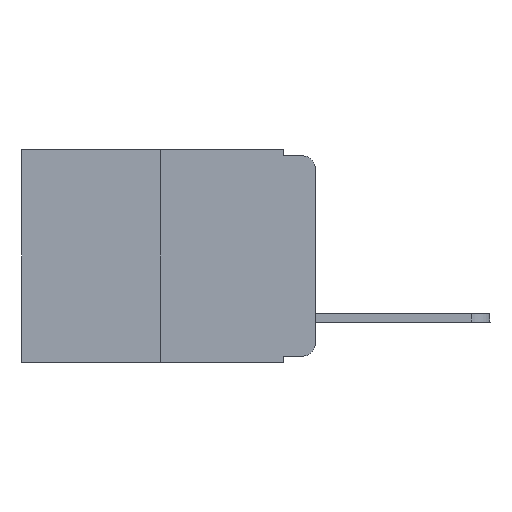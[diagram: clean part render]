
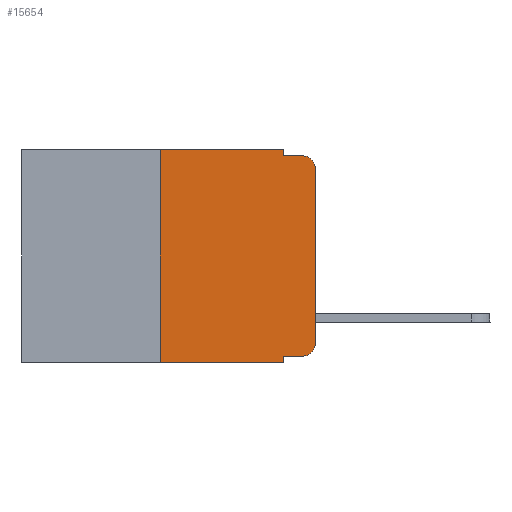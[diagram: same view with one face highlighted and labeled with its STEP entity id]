
A CAD part, left-side view. The second image highlights one B-rep face of the part: STEP entity #15654.
In plain terms, the highlighted planar face has unit normal (-1, 0, 0).
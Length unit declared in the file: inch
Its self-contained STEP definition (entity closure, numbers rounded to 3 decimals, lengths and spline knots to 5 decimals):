
#447 = DIRECTION ( 'NONE',  ( 0., -1., 0. ) ) ;
#680 = CARTESIAN_POINT ( 'NONE',  ( 0., 0.051, -0.01 ) ) ;
#931 = CARTESIAN_POINT ( 'NONE',  ( 0., 0.051, 0. ) ) ;
#967 = VECTOR ( 'NONE', #12495, 39.37008 ) ;
#1719 = LINE ( 'NONE', #7538, #967 ) ;
#1951 = ORIENTED_EDGE ( 'NONE', *, *, #15290, .T. ) ;
#2022 = VERTEX_POINT ( 'NONE', #12525 ) ;
#2119 = CARTESIAN_POINT ( 'NONE',  ( 0., 0., -0.313 ) ) ;
#2193 = VERTEX_POINT ( 'NONE', #5717 ) ;
#2201 = VERTEX_POINT ( 'NONE', #17846 ) ;
#2648 = VECTOR ( 'NONE', #9778, 39.37008 ) ;
#3068 = CARTESIAN_POINT ( 'NONE',  ( 0., 0.051, 0. ) ) ;
#3104 = DIRECTION ( 'NONE',  ( 1., 0., 0. ) ) ;
#3547 = ORIENTED_EDGE ( 'NONE', *, *, #11689, .T. ) ;
#3681 = DIRECTION ( 'NONE',  ( 0., -1., 0. ) ) ;
#4280 = VECTOR ( 'NONE', #17617, 39.37008 ) ;
#4346 = EDGE_LOOP ( 'NONE', ( #3547, #15134, #16015, #15711, #10050, #12337, #1951, #7664, #12423, #14062 ) ) ;
#4592 = AXIS2_PLACEMENT_3D ( 'NONE', #6231, #3104, #21363 ) ;
#4612 = CARTESIAN_POINT ( 'NONE',  ( 0., 0.051, -0.333 ) ) ;
#4767 = CARTESIAN_POINT ( 'NONE',  ( 0., 0., -0.03 ) ) ;
#5264 = EDGE_CURVE ( 'NONE', #10802, #16970, #11384, .T. ) ;
#5711 = DIRECTION ( 'NONE',  ( -1., 0., 0. ) ) ;
#5717 = CARTESIAN_POINT ( 'NONE',  ( 0., 0.051, -0.343 ) ) ;
#5720 = EDGE_CURVE ( 'NONE', #13088, #11283, #8902, .T. ) ;
#5899 = EDGE_CURVE ( 'NONE', #11283, #2022, #19676, .T. ) ;
#6231 = CARTESIAN_POINT ( 'NONE',  ( 0., 0.473, 0. ) ) ;
#6865 = DIRECTION ( 'NONE',  ( 0., 0., -1. ) ) ;
#7117 = CARTESIAN_POINT ( 'NONE',  ( 0., 0.473, -0.343 ) ) ;
#7363 = DIRECTION ( 'NONE',  ( 0., 0., 1. ) ) ;
#7483 = CIRCLE ( 'NONE', #19429, 0.02 ) ;
#7538 = CARTESIAN_POINT ( 'NONE',  ( 0., 0., 0. ) ) ;
#7664 = ORIENTED_EDGE ( 'NONE', *, *, #14489, .F. ) ;
#8087 = CIRCLE ( 'NONE', #9397, 0.02 ) ;
#8091 = DIRECTION ( 'NONE',  ( -1., 0., 0. ) ) ;
#8232 = VECTOR ( 'NONE', #18558, 39.37008 ) ;
#8902 = LINE ( 'NONE', #3068, #2648 ) ;
#9042 = FACE_OUTER_BOUND ( 'NONE', #4346, .T. ) ;
#9058 = VECTOR ( 'NONE', #10769, 39.37008 ) ;
#9397 = AXIS2_PLACEMENT_3D ( 'NONE', #19646, #8091, #6865 ) ;
#9632 = EDGE_CURVE ( 'NONE', #18067, #2022, #8087, .T. ) ;
#9732 = VERTEX_POINT ( 'NONE', #2119 ) ;
#9778 = DIRECTION ( 'NONE',  ( 0., 0., -1. ) ) ;
#10050 = ORIENTED_EDGE ( 'NONE', *, *, #12721, .F. ) ;
#10769 = DIRECTION ( 'NONE',  ( 0., 0., -1. ) ) ;
#10802 = VERTEX_POINT ( 'NONE', #11896 ) ;
#10995 = VECTOR ( 'NONE', #447, 39.37008 ) ;
#11052 = LINE ( 'NONE', #12459, #4280 ) ;
#11283 = VERTEX_POINT ( 'NONE', #680 ) ;
#11384 = LINE ( 'NONE', #13996, #16378 ) ;
#11689 = EDGE_CURVE ( 'NONE', #9732, #18067, #1719, .T. ) ;
#11718 = VERTEX_POINT ( 'NONE', #4612 ) ;
#11896 = CARTESIAN_POINT ( 'NONE',  ( 0., 0.25, -0.343 ) ) ;
#12204 = EDGE_CURVE ( 'NONE', #2201, #9732, #7483, .T. ) ;
#12337 = ORIENTED_EDGE ( 'NONE', *, *, #5264, .F. ) ;
#12423 = ORIENTED_EDGE ( 'NONE', *, *, #17345, .T. ) ;
#12459 = CARTESIAN_POINT ( 'NONE',  ( 0., 0.051, -0.333 ) ) ;
#12495 = DIRECTION ( 'NONE',  ( 0., 0., 1. ) ) ;
#12525 = CARTESIAN_POINT ( 'NONE',  ( 0., 0.02, -0.01 ) ) ;
#12695 = LINE ( 'NONE', #17459, #9058 ) ;
#12721 = EDGE_CURVE ( 'NONE', #16970, #13088, #21245, .T. ) ;
#13088 = VERTEX_POINT ( 'NONE', #931 ) ;
#13996 = CARTESIAN_POINT ( 'NONE',  ( 0., 0.25, 0. ) ) ;
#14019 = LINE ( 'NONE', #7117, #8232 ) ;
#14062 = ORIENTED_EDGE ( 'NONE', *, *, #12204, .T. ) ;
#14489 = EDGE_CURVE ( 'NONE', #11718, #2193, #12695, .T. ) ;
#15134 = ORIENTED_EDGE ( 'NONE', *, *, #9632, .T. ) ;
#15290 = EDGE_CURVE ( 'NONE', #10802, #2193, #14019, .T. ) ;
#15654 = ADVANCED_FACE ( 'NONE', ( #9042 ), #19811, .F. ) ;
#15711 = ORIENTED_EDGE ( 'NONE', *, *, #5720, .F. ) ;
#16015 = ORIENTED_EDGE ( 'NONE', *, *, #5899, .F. ) ;
#16378 = VECTOR ( 'NONE', #7363, 39.37008 ) ;
#16970 = VERTEX_POINT ( 'NONE', #18272 ) ;
#17345 = EDGE_CURVE ( 'NONE', #11718, #2201, #11052, .T. ) ;
#17459 = CARTESIAN_POINT ( 'NONE',  ( 0., 0.051, 0. ) ) ;
#17617 = DIRECTION ( 'NONE',  ( 0., -1., 0. ) ) ;
#17846 = CARTESIAN_POINT ( 'NONE',  ( 0., 0.02, -0.333 ) ) ;
#18067 = VERTEX_POINT ( 'NONE', #4767 ) ;
#18272 = CARTESIAN_POINT ( 'NONE',  ( 0., 0.25, 0. ) ) ;
#18558 = DIRECTION ( 'NONE',  ( 0., -1., 0. ) ) ;
#18581 = CARTESIAN_POINT ( 'NONE',  ( 0., 0.051, -0.01 ) ) ;
#18873 = VECTOR ( 'NONE', #3681, 39.37008 ) ;
#19226 = CARTESIAN_POINT ( 'NONE',  ( 0., 0.02, -0.313 ) ) ;
#19429 = AXIS2_PLACEMENT_3D ( 'NONE', #19226, #5711, #20762 ) ;
#19646 = CARTESIAN_POINT ( 'NONE',  ( 0., 0.02, -0.03 ) ) ;
#19676 = LINE ( 'NONE', #18581, #10995 ) ;
#19811 = PLANE ( 'NONE',  #4592 ) ;
#20762 = DIRECTION ( 'NONE',  ( 0., 0., -1. ) ) ;
#21245 = LINE ( 'NONE', #21494, #18873 ) ;
#21363 = DIRECTION ( 'NONE',  ( 0., 0., -1. ) ) ;
#21494 = CARTESIAN_POINT ( 'NONE',  ( 0., 0.473, 0. ) ) ;
